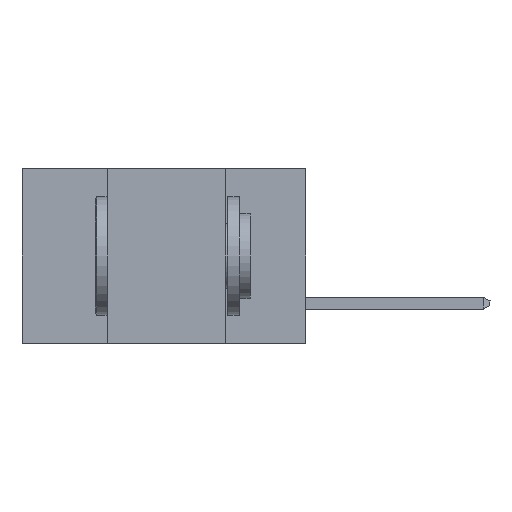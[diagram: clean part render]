
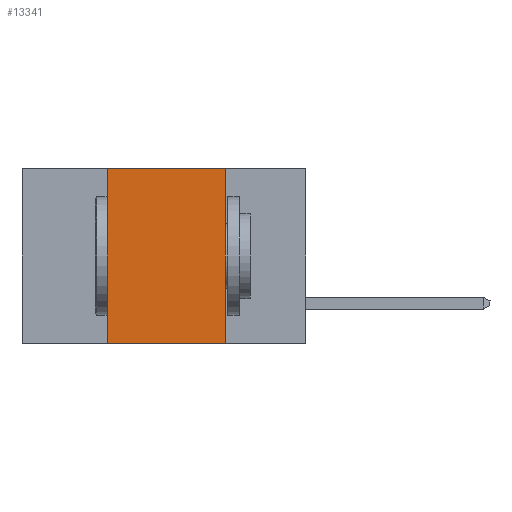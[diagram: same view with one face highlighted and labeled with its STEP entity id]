
A CAD part, left-side view. The second image highlights one B-rep face of the part: STEP entity #13341.
In plain terms, the highlighted planar face has unit normal (-1, 0, 0).
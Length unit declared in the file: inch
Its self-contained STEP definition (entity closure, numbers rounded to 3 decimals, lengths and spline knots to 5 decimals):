
#55 = DIRECTION ( 'NONE',  ( 0., 0., 1. ) ) ;
#271 = VERTEX_POINT ( 'NONE', #2174 ) ;
#665 = ORIENTED_EDGE ( 'NONE', *, *, #14474, .F. ) ;
#742 = VECTOR ( 'NONE', #17465, 39.37008 ) ;
#827 = VERTEX_POINT ( 'NONE', #16253 ) ;
#848 = CARTESIAN_POINT ( 'NONE',  ( 0., 0.6, 0. ) ) ;
#1408 = CARTESIAN_POINT ( 'NONE',  ( 0., 0.42, 0. ) ) ;
#1628 = CARTESIAN_POINT ( 'NONE',  ( 0., 0.42, 0. ) ) ;
#1905 = CARTESIAN_POINT ( 'NONE',  ( 0., 0.42, -0.37 ) ) ;
#2112 = DIRECTION ( 'NONE',  ( 0., 0., -1. ) ) ;
#2174 = CARTESIAN_POINT ( 'NONE',  ( 0., 0.17, -0.37 ) ) ;
#2729 = DIRECTION ( 'NONE',  ( 1., 0., 0. ) ) ;
#3751 = LINE ( 'NONE', #848, #742 ) ;
#5252 = PLANE ( 'NONE',  #17469 ) ;
#5281 = VECTOR ( 'NONE', #14512, 39.37008 ) ;
#6024 = EDGE_CURVE ( 'NONE', #13621, #271, #14800, .T. ) ;
#6256 = ORIENTED_EDGE ( 'NONE', *, *, #14350, .F. ) ;
#6491 = LINE ( 'NONE', #1628, #7388 ) ;
#6895 = DIRECTION ( 'NONE',  ( 0., 0., -1. ) ) ;
#7388 = VECTOR ( 'NONE', #55, 39.37008 ) ;
#8632 = LINE ( 'NONE', #12693, #15301 ) ;
#8687 = ORIENTED_EDGE ( 'NONE', *, *, #6024, .T. ) ;
#9110 = EDGE_CURVE ( 'NONE', #13621, #15867, #6491, .T. ) ;
#9487 = CARTESIAN_POINT ( 'NONE',  ( 0., 0.6, 0. ) ) ;
#10317 = FACE_OUTER_BOUND ( 'NONE', #11281, .T. ) ;
#11281 = EDGE_LOOP ( 'NONE', ( #665, #6256, #15205, #8687 ) ) ;
#12693 = CARTESIAN_POINT ( 'NONE',  ( 0., 0.17, 0. ) ) ;
#13341 = ADVANCED_FACE ( 'NONE', ( #10317 ), #5252, .F. ) ;
#13621 = VERTEX_POINT ( 'NONE', #1905 ) ;
#14350 = EDGE_CURVE ( 'NONE', #15867, #827, #3751, .T. ) ;
#14457 = CARTESIAN_POINT ( 'NONE',  ( 0., 0.6, -0.37 ) ) ;
#14474 = EDGE_CURVE ( 'NONE', #827, #271, #8632, .T. ) ;
#14512 = DIRECTION ( 'NONE',  ( 0., -1., 0. ) ) ;
#14800 = LINE ( 'NONE', #14457, #5281 ) ;
#15205 = ORIENTED_EDGE ( 'NONE', *, *, #9110, .F. ) ;
#15301 = VECTOR ( 'NONE', #2112, 39.37008 ) ;
#15867 = VERTEX_POINT ( 'NONE', #1408 ) ;
#16253 = CARTESIAN_POINT ( 'NONE',  ( 0., 0.17, 0. ) ) ;
#17465 = DIRECTION ( 'NONE',  ( 0., -1., 0. ) ) ;
#17469 = AXIS2_PLACEMENT_3D ( 'NONE', #9487, #2729, #6895 ) ;
